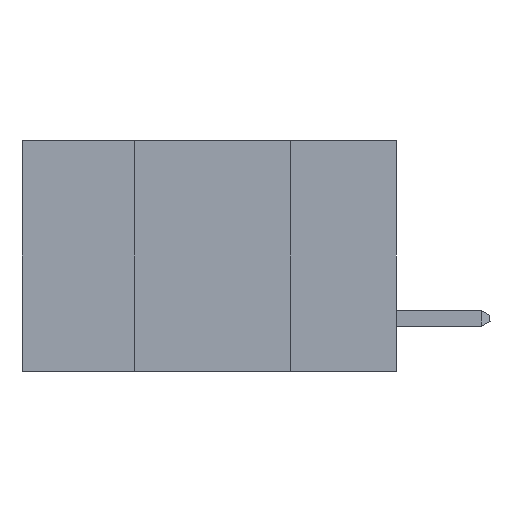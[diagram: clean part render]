
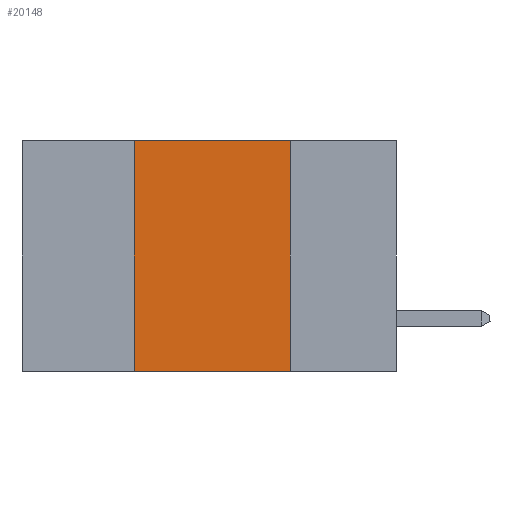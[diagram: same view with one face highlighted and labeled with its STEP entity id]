
A CAD part, left-side view. The second image highlights one B-rep face of the part: STEP entity #20148.
In plain terms, the highlighted planar face has unit normal (-1, 0, 0).
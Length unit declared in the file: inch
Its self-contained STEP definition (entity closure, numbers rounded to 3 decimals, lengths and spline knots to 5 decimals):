
#455 = DIRECTION ( 'NONE',  ( 0., 0., -1. ) ) ;
#608 = DIRECTION ( 'NONE',  ( 0., 0., -1. ) ) ;
#2570 = DIRECTION ( 'NONE',  ( 1., 0., 0. ) ) ;
#2853 = CARTESIAN_POINT ( 'NONE',  ( 0., 0.42, -0.37 ) ) ;
#3636 = VERTEX_POINT ( 'NONE', #20351 ) ;
#3895 = ORIENTED_EDGE ( 'NONE', *, *, #8453, .T. ) ;
#4581 = VECTOR ( 'NONE', #7424, 39.37008 ) ;
#4586 = DIRECTION ( 'NONE',  ( 0., 0., 1. ) ) ;
#6368 = CARTESIAN_POINT ( 'NONE',  ( 0., 0.42, 0. ) ) ;
#6964 = VECTOR ( 'NONE', #4586, 39.37008 ) ;
#7027 = VECTOR ( 'NONE', #11232, 39.37008 ) ;
#7305 = CARTESIAN_POINT ( 'NONE',  ( 0., 0.6, -0.37 ) ) ;
#7424 = DIRECTION ( 'NONE',  ( 0., -1., 0. ) ) ;
#7716 = FACE_OUTER_BOUND ( 'NONE', #19800, .T. ) ;
#8453 = EDGE_CURVE ( 'NONE', #11174, #3636, #19252, .T. ) ;
#10498 = EDGE_CURVE ( 'NONE', #11174, #18338, #11541, .T. ) ;
#11174 = VERTEX_POINT ( 'NONE', #2853 ) ;
#11232 = DIRECTION ( 'NONE',  ( 0., -1., 0. ) ) ;
#11541 = LINE ( 'NONE', #6368, #6964 ) ;
#14632 = AXIS2_PLACEMENT_3D ( 'NONE', #23810, #2570, #608 ) ;
#14984 = LINE ( 'NONE', #16857, #4581 ) ;
#16290 = EDGE_CURVE ( 'NONE', #18338, #22687, #14984, .T. ) ;
#16759 = VECTOR ( 'NONE', #455, 39.37008 ) ;
#16839 = EDGE_CURVE ( 'NONE', #22687, #3636, #17369, .T. ) ;
#16857 = CARTESIAN_POINT ( 'NONE',  ( 0., 0.6, 0. ) ) ;
#17369 = LINE ( 'NONE', #21973, #16759 ) ;
#18338 = VERTEX_POINT ( 'NONE', #21626 ) ;
#19252 = LINE ( 'NONE', #7305, #7027 ) ;
#19800 = EDGE_LOOP ( 'NONE', ( #21265, #23388, #23373, #3895 ) ) ;
#20148 = ADVANCED_FACE ( 'NONE', ( #7716 ), #21719, .F. ) ;
#20351 = CARTESIAN_POINT ( 'NONE',  ( 0., 0.17, -0.37 ) ) ;
#21265 = ORIENTED_EDGE ( 'NONE', *, *, #16839, .F. ) ;
#21626 = CARTESIAN_POINT ( 'NONE',  ( 0., 0.42, 0. ) ) ;
#21719 = PLANE ( 'NONE',  #14632 ) ;
#21973 = CARTESIAN_POINT ( 'NONE',  ( 0., 0.17, 0. ) ) ;
#22687 = VERTEX_POINT ( 'NONE', #23146 ) ;
#23146 = CARTESIAN_POINT ( 'NONE',  ( 0., 0.17, 0. ) ) ;
#23373 = ORIENTED_EDGE ( 'NONE', *, *, #10498, .F. ) ;
#23388 = ORIENTED_EDGE ( 'NONE', *, *, #16290, .F. ) ;
#23810 = CARTESIAN_POINT ( 'NONE',  ( 0., 0.6, 0. ) ) ;
